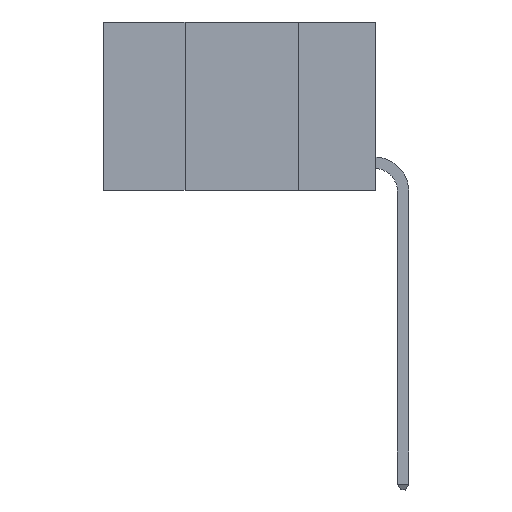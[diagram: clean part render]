
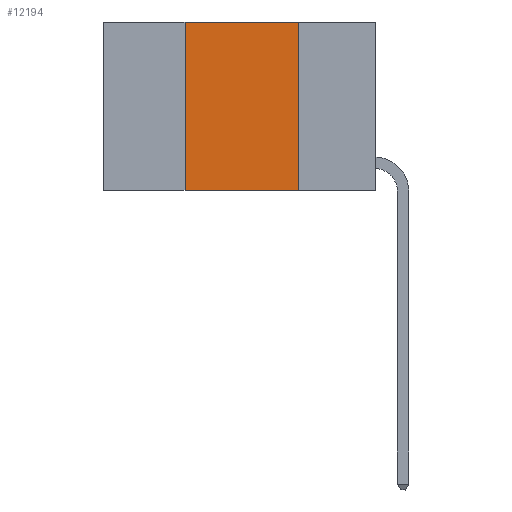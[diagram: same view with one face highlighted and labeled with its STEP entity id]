
A CAD part, left-side view. The second image highlights one B-rep face of the part: STEP entity #12194.
In plain terms, the highlighted planar face has unit normal (-1, 0, 0).
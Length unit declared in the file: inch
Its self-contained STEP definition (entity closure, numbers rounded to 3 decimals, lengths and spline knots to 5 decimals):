
#945 = DIRECTION ( 'NONE',  ( 0., 0., 1. ) ) ;
#1447 = ORIENTED_EDGE ( 'NONE', *, *, #13481, .F. ) ;
#1591 = CARTESIAN_POINT ( 'NONE',  ( 0., 0.6, 0. ) ) ;
#2483 = VECTOR ( 'NONE', #9810, 39.37008 ) ;
#2634 = ORIENTED_EDGE ( 'NONE', *, *, #5815, .T. ) ;
#3519 = ORIENTED_EDGE ( 'NONE', *, *, #7124, .F. ) ;
#3585 = FACE_OUTER_BOUND ( 'NONE', #15103, .T. ) ;
#4039 = CARTESIAN_POINT ( 'NONE',  ( 0., 0.17, -0.37 ) ) ;
#4170 = ORIENTED_EDGE ( 'NONE', *, *, #7328, .F. ) ;
#4459 = PLANE ( 'NONE',  #12944 ) ;
#5815 = EDGE_CURVE ( 'NONE', #7370, #11539, #6304, .T. ) ;
#5889 = DIRECTION ( 'NONE',  ( 0., 0., -1. ) ) ;
#6304 = LINE ( 'NONE', #16102, #13631 ) ;
#7124 = EDGE_CURVE ( 'NONE', #7370, #7579, #9671, .T. ) ;
#7328 = EDGE_CURVE ( 'NONE', #7579, #9436, #13143, .T. ) ;
#7370 = VERTEX_POINT ( 'NONE', #8560 ) ;
#7579 = VERTEX_POINT ( 'NONE', #7735 ) ;
#7735 = CARTESIAN_POINT ( 'NONE',  ( 0., 0.42, 0. ) ) ;
#7851 = DIRECTION ( 'NONE',  ( 0., -1., 0. ) ) ;
#8444 = CARTESIAN_POINT ( 'NONE',  ( 0., 0.6, 0. ) ) ;
#8560 = CARTESIAN_POINT ( 'NONE',  ( 0., 0.42, -0.37 ) ) ;
#8648 = DIRECTION ( 'NONE',  ( 0., 0., -1. ) ) ;
#9239 = VECTOR ( 'NONE', #945, 39.37008 ) ;
#9276 = CARTESIAN_POINT ( 'NONE',  ( 0., 0.17, 0. ) ) ;
#9436 = VERTEX_POINT ( 'NONE', #9276 ) ;
#9671 = LINE ( 'NONE', #12164, #9239 ) ;
#9810 = DIRECTION ( 'NONE',  ( 0., -1., 0. ) ) ;
#11539 = VERTEX_POINT ( 'NONE', #4039 ) ;
#12164 = CARTESIAN_POINT ( 'NONE',  ( 0., 0.42, 0. ) ) ;
#12194 = ADVANCED_FACE ( 'NONE', ( #3585 ), #4459, .F. ) ;
#12944 = AXIS2_PLACEMENT_3D ( 'NONE', #1591, #14133, #5889 ) ;
#13143 = LINE ( 'NONE', #8444, #2483 ) ;
#13294 = VECTOR ( 'NONE', #8648, 39.37008 ) ;
#13481 = EDGE_CURVE ( 'NONE', #9436, #11539, #13709, .T. ) ;
#13631 = VECTOR ( 'NONE', #7851, 39.37008 ) ;
#13709 = LINE ( 'NONE', #16933, #13294 ) ;
#14133 = DIRECTION ( 'NONE',  ( 1., 0., 0. ) ) ;
#15103 = EDGE_LOOP ( 'NONE', ( #1447, #4170, #3519, #2634 ) ) ;
#16102 = CARTESIAN_POINT ( 'NONE',  ( 0., 0.6, -0.37 ) ) ;
#16933 = CARTESIAN_POINT ( 'NONE',  ( 0., 0.17, 0. ) ) ;
